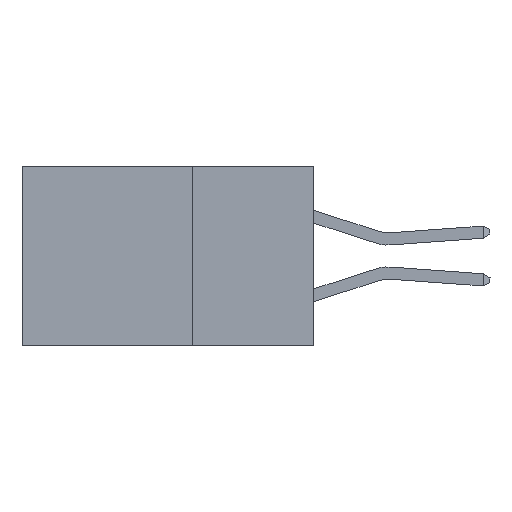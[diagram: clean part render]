
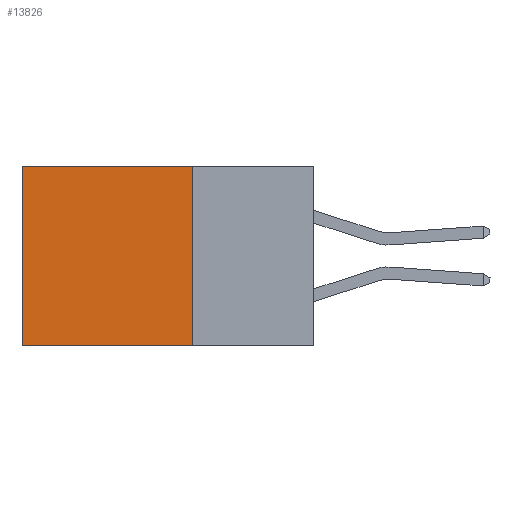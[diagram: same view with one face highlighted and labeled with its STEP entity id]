
A CAD part, left-side view. The second image highlights one B-rep face of the part: STEP entity #13826.
In plain terms, the highlighted planar face has unit normal (-1, 0, 0).
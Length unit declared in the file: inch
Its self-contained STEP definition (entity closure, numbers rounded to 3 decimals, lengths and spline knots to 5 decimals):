
#1235 = CARTESIAN_POINT ( 'NONE',  ( 0.2875, 0.25, 0. ) ) ;
#1598 = PLANE ( 'NONE',  #5657 ) ;
#1901 = EDGE_CURVE ( 'NONE', #15856, #14536, #5778, .T. ) ;
#2462 = CARTESIAN_POINT ( 'NONE',  ( 0.2875, 0.6, 0. ) ) ;
#3308 = CARTESIAN_POINT ( 'NONE',  ( 0.2875, 0.25, 0. ) ) ;
#3393 = CARTESIAN_POINT ( 'NONE',  ( 0.2875, 0.25, 0. ) ) ;
#3490 = DIRECTION ( 'NONE',  ( 1., 0., 0. ) ) ;
#3744 = ORIENTED_EDGE ( 'NONE', *, *, #20400, .F. ) ;
#5325 = EDGE_CURVE ( 'NONE', #14536, #8413, #16900, .T. ) ;
#5657 = AXIS2_PLACEMENT_3D ( 'NONE', #3308, #3490, #24031 ) ;
#5778 = LINE ( 'NONE', #3393, #18845 ) ;
#5801 = CARTESIAN_POINT ( 'NONE',  ( 0.2875, 0.6, 0. ) ) ;
#6552 = DIRECTION ( 'NONE',  ( 0., 0., -1. ) ) ;
#7991 = CARTESIAN_POINT ( 'NONE',  ( 0.2875, 0.25, -0.37 ) ) ;
#8375 = CARTESIAN_POINT ( 'NONE',  ( 0.2875, 0.25, 0. ) ) ;
#8382 = ORIENTED_EDGE ( 'NONE', *, *, #1901, .T. ) ;
#8413 = VERTEX_POINT ( 'NONE', #8489 ) ;
#8489 = CARTESIAN_POINT ( 'NONE',  ( 0.2875, 0.6, -0.37 ) ) ;
#9572 = DIRECTION ( 'NONE',  ( 0., 1., 0. ) ) ;
#9829 = EDGE_LOOP ( 'NONE', ( #14159, #3744, #17480, #8382 ) ) ;
#10152 = LINE ( 'NONE', #22828, #23883 ) ;
#11497 = VECTOR ( 'NONE', #13036, 39.37008 ) ;
#12923 = LINE ( 'NONE', #8375, #21164 ) ;
#13036 = DIRECTION ( 'NONE',  ( 0., 0., -1. ) ) ;
#13826 = ADVANCED_FACE ( 'NONE', ( #20928 ), #1598, .F. ) ;
#14159 = ORIENTED_EDGE ( 'NONE', *, *, #5325, .T. ) ;
#14536 = VERTEX_POINT ( 'NONE', #5801 ) ;
#15856 = VERTEX_POINT ( 'NONE', #1235 ) ;
#16900 = LINE ( 'NONE', #2462, #11497 ) ;
#17035 = VERTEX_POINT ( 'NONE', #7991 ) ;
#17480 = ORIENTED_EDGE ( 'NONE', *, *, #25706, .F. ) ;
#18845 = VECTOR ( 'NONE', #9572, 39.37008 ) ;
#20400 = EDGE_CURVE ( 'NONE', #17035, #8413, #10152, .T. ) ;
#20592 = DIRECTION ( 'NONE',  ( 0., 1., 0. ) ) ;
#20928 = FACE_OUTER_BOUND ( 'NONE', #9829, .T. ) ;
#21164 = VECTOR ( 'NONE', #6552, 39.37008 ) ;
#22828 = CARTESIAN_POINT ( 'NONE',  ( 0.2875, 0.25, -0.37 ) ) ;
#23883 = VECTOR ( 'NONE', #20592, 39.37008 ) ;
#24031 = DIRECTION ( 'NONE',  ( 0., 0., -1. ) ) ;
#25706 = EDGE_CURVE ( 'NONE', #15856, #17035, #12923, .T. ) ;
